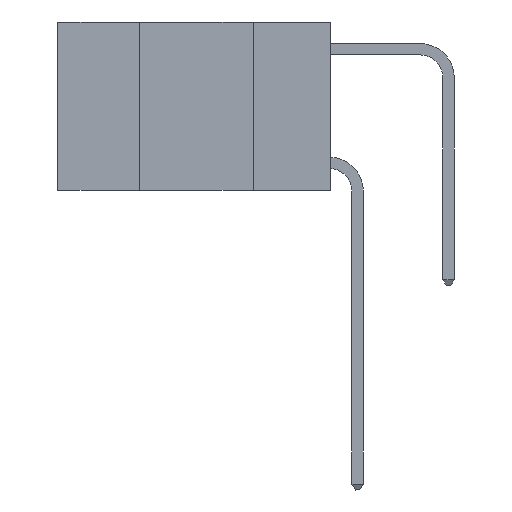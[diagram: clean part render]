
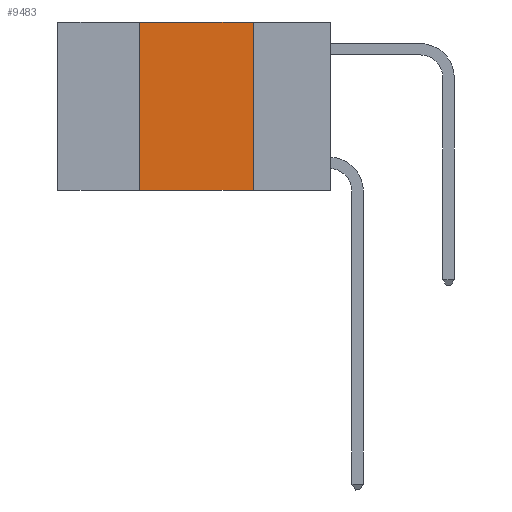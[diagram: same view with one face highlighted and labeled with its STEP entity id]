
A CAD part, left-side view. The second image highlights one B-rep face of the part: STEP entity #9483.
In plain terms, the highlighted planar face has unit normal (-1, 0, 0).
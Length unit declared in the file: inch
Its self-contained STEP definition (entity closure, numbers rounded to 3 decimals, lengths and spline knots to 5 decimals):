
#6315 = VERTEX_POINT ( 'NONE', #25676 ) ;
#7684 = ORIENTED_EDGE ( 'NONE', *, *, #29120, .F. ) ;
#8239 = DIRECTION ( 'NONE',  ( 0., 0., 1. ) ) ;
#9483 = ADVANCED_FACE ( 'NONE', ( #18712 ), #28477, .F. ) ;
#10080 = VECTOR ( 'NONE', #8239, 39.37008 ) ;
#12376 = DIRECTION ( 'NONE',  ( 1., 0., 0. ) ) ;
#12690 = ORIENTED_EDGE ( 'NONE', *, *, #23885, .T. ) ;
#14031 = VECTOR ( 'NONE', #20500, 39.37008 ) ;
#15975 = VERTEX_POINT ( 'NONE', #26393 ) ;
#16053 = VECTOR ( 'NONE', #22033, 39.37008 ) ;
#16612 = CARTESIAN_POINT ( 'NONE',  ( 0., 0.17, 0. ) ) ;
#17219 = LINE ( 'NONE', #29606, #10080 ) ;
#17758 = CARTESIAN_POINT ( 'NONE',  ( 0., 0.6, 0. ) ) ;
#18712 = FACE_OUTER_BOUND ( 'NONE', #29607, .T. ) ;
#20500 = DIRECTION ( 'NONE',  ( 0., -1., 0. ) ) ;
#22033 = DIRECTION ( 'NONE',  ( 0., 0., -1. ) ) ;
#22359 = CARTESIAN_POINT ( 'NONE',  ( 0., 0.42, 0. ) ) ;
#23224 = LINE ( 'NONE', #16612, #16053 ) ;
#23885 = EDGE_CURVE ( 'NONE', #6315, #15975, #28522, .T. ) ;
#25676 = CARTESIAN_POINT ( 'NONE',  ( 0., 0.42, -0.37 ) ) ;
#25794 = CARTESIAN_POINT ( 'NONE',  ( 0., 0.6, 0. ) ) ;
#26370 = EDGE_CURVE ( 'NONE', #27861, #33901, #28316, .T. ) ;
#26393 = CARTESIAN_POINT ( 'NONE',  ( 0., 0.17, -0.37 ) ) ;
#26811 = DIRECTION ( 'NONE',  ( 0., -1., 0. ) ) ;
#27698 = VECTOR ( 'NONE', #26811, 39.37008 ) ;
#27760 = ORIENTED_EDGE ( 'NONE', *, *, #33523, .F. ) ;
#27861 = VERTEX_POINT ( 'NONE', #22359 ) ;
#28316 = LINE ( 'NONE', #17758, #14031 ) ;
#28477 = PLANE ( 'NONE',  #29369 ) ;
#28522 = LINE ( 'NONE', #32065, #27698 ) ;
#29120 = EDGE_CURVE ( 'NONE', #33901, #15975, #23224, .T. ) ;
#29369 = AXIS2_PLACEMENT_3D ( 'NONE', #25794, #12376, #31171 ) ;
#29606 = CARTESIAN_POINT ( 'NONE',  ( 0., 0.42, 0. ) ) ;
#29607 = EDGE_LOOP ( 'NONE', ( #7684, #32794, #27760, #12690 ) ) ;
#31121 = CARTESIAN_POINT ( 'NONE',  ( 0., 0.17, 0. ) ) ;
#31171 = DIRECTION ( 'NONE',  ( 0., 0., -1. ) ) ;
#32065 = CARTESIAN_POINT ( 'NONE',  ( 0., 0.6, -0.37 ) ) ;
#32794 = ORIENTED_EDGE ( 'NONE', *, *, #26370, .F. ) ;
#33523 = EDGE_CURVE ( 'NONE', #6315, #27861, #17219, .T. ) ;
#33901 = VERTEX_POINT ( 'NONE', #31121 ) ;
